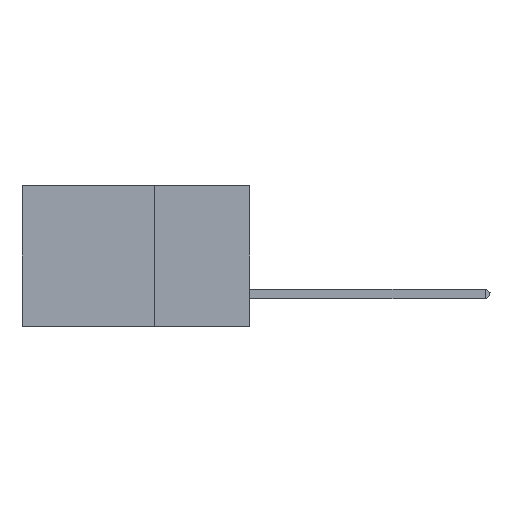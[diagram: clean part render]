
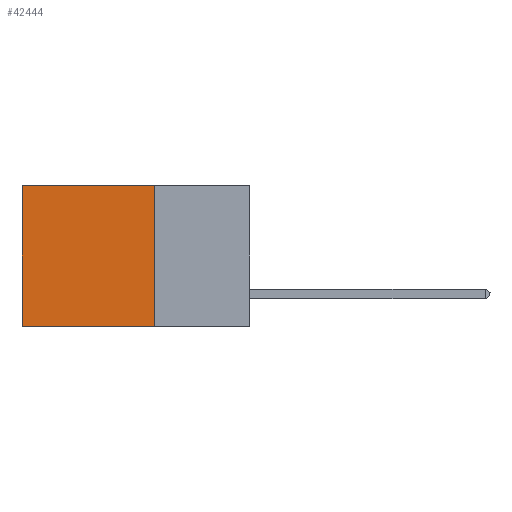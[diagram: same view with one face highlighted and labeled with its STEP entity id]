
A CAD part, left-side view. The second image highlights one B-rep face of the part: STEP entity #42444.
In plain terms, the highlighted planar face has unit normal (-1, 0, 0).
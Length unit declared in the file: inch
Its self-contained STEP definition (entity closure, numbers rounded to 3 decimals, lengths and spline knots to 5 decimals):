
#100 = DIRECTION ( 'NONE',  ( 0., 0., -1. ) ) ;
#221 = EDGE_CURVE ( 'NONE', #33045, #31564, #24940, .T. ) ;
#996 = EDGE_CURVE ( 'NONE', #15415, #6242, #41388, .T. ) ;
#3918 = CARTESIAN_POINT ( 'NONE',  ( 0.2875, 0.6, -0.37 ) ) ;
#6242 = VERTEX_POINT ( 'NONE', #3918 ) ;
#7189 = DIRECTION ( 'NONE',  ( 0., 1., 0. ) ) ;
#8391 = VECTOR ( 'NONE', #38539, 39.37008 ) ;
#8644 = EDGE_LOOP ( 'NONE', ( #10415, #21377, #34107, #19212 ) ) ;
#10002 = VECTOR ( 'NONE', #100, 39.37008 ) ;
#10415 = ORIENTED_EDGE ( 'NONE', *, *, #26961, .T. ) ;
#13580 = LINE ( 'NONE', #16634, #10002 ) ;
#14281 = CARTESIAN_POINT ( 'NONE',  ( 0.2875, 0.6, 0. ) ) ;
#14709 = DIRECTION ( 'NONE',  ( 0., 0., -1. ) ) ;
#15043 = VECTOR ( 'NONE', #7189, 39.37008 ) ;
#15415 = VERTEX_POINT ( 'NONE', #19923 ) ;
#16634 = CARTESIAN_POINT ( 'NONE',  ( 0.2875, 0.25, 0. ) ) ;
#17271 = CARTESIAN_POINT ( 'NONE',  ( 0.2875, 0.25, -0.37 ) ) ;
#19212 = ORIENTED_EDGE ( 'NONE', *, *, #221, .T. ) ;
#19923 = CARTESIAN_POINT ( 'NONE',  ( 0.2875, 0.25, -0.37 ) ) ;
#21377 = ORIENTED_EDGE ( 'NONE', *, *, #996, .F. ) ;
#24667 = DIRECTION ( 'NONE',  ( 0., 0., -1. ) ) ;
#24940 = LINE ( 'NONE', #25587, #8391 ) ;
#25587 = CARTESIAN_POINT ( 'NONE',  ( 0.2875, 0.25, 0. ) ) ;
#25787 = CARTESIAN_POINT ( 'NONE',  ( 0.2875, 0.6, 0. ) ) ;
#26961 = EDGE_CURVE ( 'NONE', #31564, #6242, #27180, .T. ) ;
#27180 = LINE ( 'NONE', #14281, #30272 ) ;
#27680 = DIRECTION ( 'NONE',  ( 1., 0., 0. ) ) ;
#28194 = CARTESIAN_POINT ( 'NONE',  ( 0.2875, 0.25, 0. ) ) ;
#30272 = VECTOR ( 'NONE', #14709, 39.37008 ) ;
#30650 = AXIS2_PLACEMENT_3D ( 'NONE', #41368, #27680, #24667 ) ;
#31416 = PLANE ( 'NONE',  #30650 ) ;
#31564 = VERTEX_POINT ( 'NONE', #25787 ) ;
#33045 = VERTEX_POINT ( 'NONE', #28194 ) ;
#34107 = ORIENTED_EDGE ( 'NONE', *, *, #40047, .F. ) ;
#38539 = DIRECTION ( 'NONE',  ( 0., 1., 0. ) ) ;
#39971 = FACE_OUTER_BOUND ( 'NONE', #8644, .T. ) ;
#40047 = EDGE_CURVE ( 'NONE', #33045, #15415, #13580, .T. ) ;
#41368 = CARTESIAN_POINT ( 'NONE',  ( 0.2875, 0.25, 0. ) ) ;
#41388 = LINE ( 'NONE', #17271, #15043 ) ;
#42444 = ADVANCED_FACE ( 'NONE', ( #39971 ), #31416, .F. ) ;
